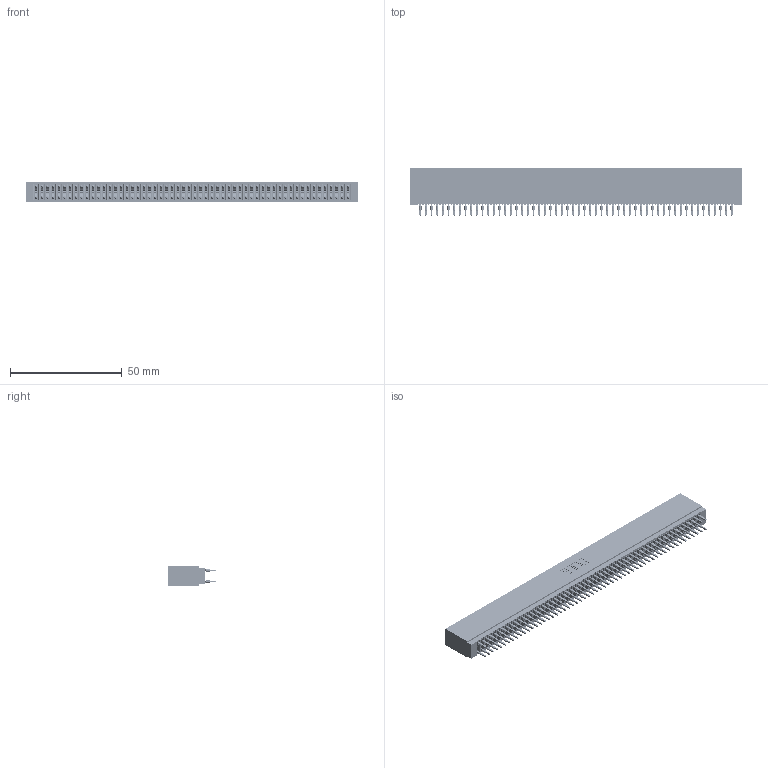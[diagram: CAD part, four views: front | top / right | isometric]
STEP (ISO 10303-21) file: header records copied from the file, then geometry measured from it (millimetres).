
FILE_DESCRIPTION (( 'STEP AP203' ), '1' );
FILE_NAME ('745-112-520-201.STEP', '2026-02-27T00:27:17', ( '' ), ( '' ), 'SwSTEP 2.0', 'SolidWorks 2023', '' );
FILE_SCHEMA (( 'CONFIG_CONTROL_DESIGN' ));
Length unit declared in the file: millimetre
Products named in the file (3): 745 Part_Insulator Option - 01; 745-112-520-201; 745-292-001_520
Assembly tree (113 placements, depth 2):
  745-112-520-201
    745 Part_Insulator Option - 01
    745-292-001_520  x112
Bounding box: 148.84 x 21.22 x 8.89 mm (x, y, z)
Volume: 13226.7 mm3; surface area: 26694.9 mm2
Topology: 113 solids, 113 shells, 10119 faces, 27194 edges, 17084 vertices
Faces by surface type: plane 5207, bspline 2240, cylinder 2000, torus 672
Entity records: 92366 total; most frequent: CARTESIAN_POINT 16519, ORIENTED_EDGE 15982, DIRECTION 13949, EDGE_CURVE 7991, LINE 7473, VECTOR 7473, VERTEX_POINT 5096, AXIS2_PLACEMENT_3D 3238
